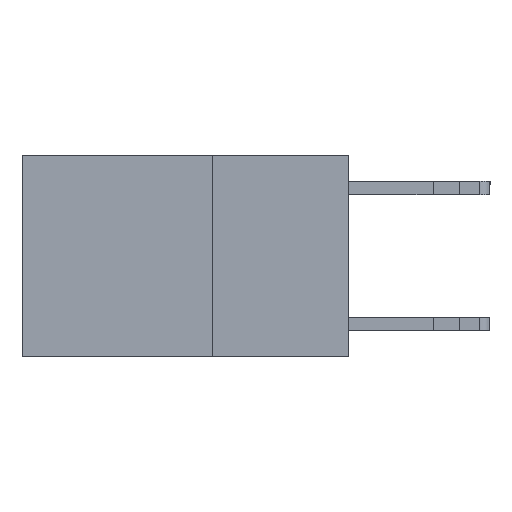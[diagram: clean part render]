
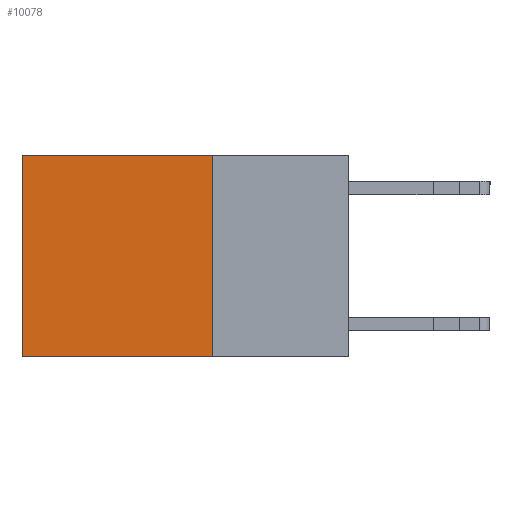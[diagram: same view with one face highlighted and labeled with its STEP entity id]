
A CAD part, left-side view. The second image highlights one B-rep face of the part: STEP entity #10078.
In plain terms, the highlighted planar face has unit normal (-1, 0, 0).
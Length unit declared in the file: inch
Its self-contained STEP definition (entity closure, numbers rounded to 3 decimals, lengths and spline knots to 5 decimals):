
#155 = LINE ( 'NONE', #8424, #5135 ) ;
#678 = CARTESIAN_POINT ( 'NONE',  ( 0.2625, 0.6, 0. ) ) ;
#1045 = CARTESIAN_POINT ( 'NONE',  ( 0.2625, 0.6, 0. ) ) ;
#1231 = AXIS2_PLACEMENT_3D ( 'NONE', #7427, #6344, #5389 ) ;
#1885 = CARTESIAN_POINT ( 'NONE',  ( 0.2625, 0.6, -0.37 ) ) ;
#1963 = VECTOR ( 'NONE', #4152, 39.37008 ) ;
#2033 = DIRECTION ( 'NONE',  ( 0., 0., -1. ) ) ;
#2176 = LINE ( 'NONE', #1045, #1963 ) ;
#3469 = EDGE_CURVE ( 'NONE', #5976, #13116, #155, .T. ) ;
#3717 = LINE ( 'NONE', #9758, #5762 ) ;
#3810 = VERTEX_POINT ( 'NONE', #678 ) ;
#4152 = DIRECTION ( 'NONE',  ( 0., 0., -1. ) ) ;
#4289 = ORIENTED_EDGE ( 'NONE', *, *, #9766, .F. ) ;
#4324 = ORIENTED_EDGE ( 'NONE', *, *, #10917, .T. ) ;
#4635 = DIRECTION ( 'NONE',  ( 0., 1., 0. ) ) ;
#5135 = VECTOR ( 'NONE', #2033, 39.37008 ) ;
#5174 = VERTEX_POINT ( 'NONE', #1885 ) ;
#5389 = DIRECTION ( 'NONE',  ( 0., 0., -1. ) ) ;
#5762 = VECTOR ( 'NONE', #6621, 39.37008 ) ;
#5976 = VERTEX_POINT ( 'NONE', #11076 ) ;
#6344 = DIRECTION ( 'NONE',  ( 1., 0., 0. ) ) ;
#6597 = EDGE_LOOP ( 'NONE', ( #4324, #4289, #10467, #11213 ) ) ;
#6621 = DIRECTION ( 'NONE',  ( 0., 1., 0. ) ) ;
#7362 = FACE_OUTER_BOUND ( 'NONE', #6597, .T. ) ;
#7427 = CARTESIAN_POINT ( 'NONE',  ( 0.2625, 0.25, 0. ) ) ;
#7544 = EDGE_CURVE ( 'NONE', #5976, #3810, #9677, .T. ) ;
#8424 = CARTESIAN_POINT ( 'NONE',  ( 0.2625, 0.25, 0. ) ) ;
#8525 = PLANE ( 'NONE',  #1231 ) ;
#8573 = CARTESIAN_POINT ( 'NONE',  ( 0.2625, 0.25, -0.37 ) ) ;
#9677 = LINE ( 'NONE', #10625, #11092 ) ;
#9758 = CARTESIAN_POINT ( 'NONE',  ( 0.2625, 0.25, -0.37 ) ) ;
#9766 = EDGE_CURVE ( 'NONE', #13116, #5174, #3717, .T. ) ;
#10078 = ADVANCED_FACE ( 'NONE', ( #7362 ), #8525, .F. ) ;
#10467 = ORIENTED_EDGE ( 'NONE', *, *, #3469, .F. ) ;
#10625 = CARTESIAN_POINT ( 'NONE',  ( 0.2625, 0.25, 0. ) ) ;
#10917 = EDGE_CURVE ( 'NONE', #3810, #5174, #2176, .T. ) ;
#11076 = CARTESIAN_POINT ( 'NONE',  ( 0.2625, 0.25, 0. ) ) ;
#11092 = VECTOR ( 'NONE', #4635, 39.37008 ) ;
#11213 = ORIENTED_EDGE ( 'NONE', *, *, #7544, .T. ) ;
#13116 = VERTEX_POINT ( 'NONE', #8573 ) ;
